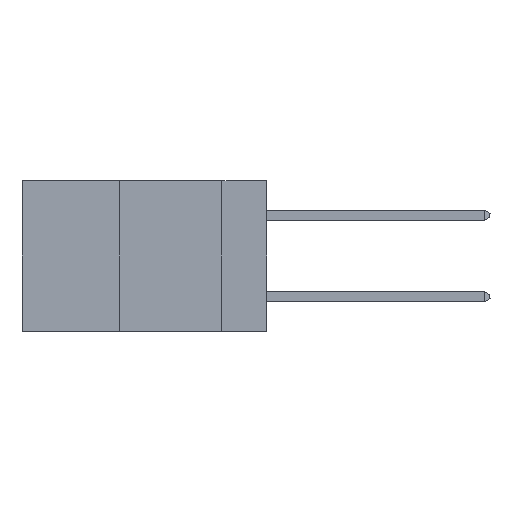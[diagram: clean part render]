
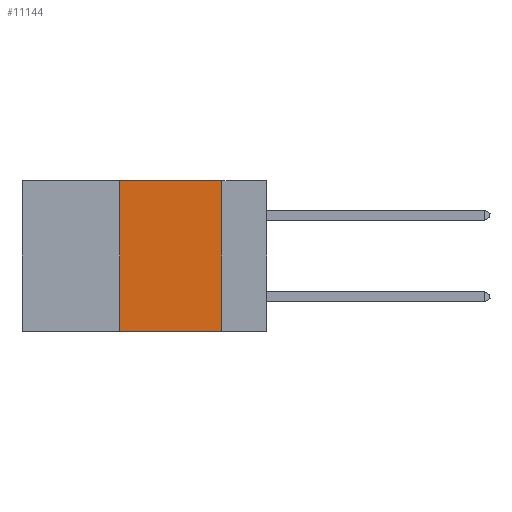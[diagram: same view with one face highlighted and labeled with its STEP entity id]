
A CAD part, left-side view. The second image highlights one B-rep face of the part: STEP entity #11144.
In plain terms, the highlighted planar face has unit normal (-1, 0, 0).
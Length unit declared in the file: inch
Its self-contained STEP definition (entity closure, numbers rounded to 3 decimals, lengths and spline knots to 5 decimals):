
#583 = DIRECTION ( 'NONE',  ( 0., 0., -1. ) ) ;
#2039 = LINE ( 'NONE', #22067, #15603 ) ;
#2174 = DIRECTION ( 'NONE',  ( 1., 0., 0. ) ) ;
#2341 = CARTESIAN_POINT ( 'NONE',  ( 0., 0.11, 0. ) ) ;
#3543 = AXIS2_PLACEMENT_3D ( 'NONE', #13882, #2174, #8664 ) ;
#5742 = LINE ( 'NONE', #2341, #22319 ) ;
#6015 = DIRECTION ( 'NONE',  ( 0., -1., 0. ) ) ;
#6436 = DIRECTION ( 'NONE',  ( 0., 0., 1. ) ) ;
#7558 = EDGE_CURVE ( 'NONE', #18047, #16710, #2039, .T. ) ;
#8325 = CARTESIAN_POINT ( 'NONE',  ( 0., 0.36, 0. ) ) ;
#8664 = DIRECTION ( 'NONE',  ( 0., 0., -1. ) ) ;
#9633 = PLANE ( 'NONE',  #3543 ) ;
#11144 = ADVANCED_FACE ( 'NONE', ( #20421 ), #9633, .F. ) ;
#12437 = DIRECTION ( 'NONE',  ( 0., -1., 0. ) ) ;
#13456 = LINE ( 'NONE', #8325, #18018 ) ;
#13805 = LINE ( 'NONE', #24127, #24475 ) ;
#13882 = CARTESIAN_POINT ( 'NONE',  ( 0., 0.6, 0. ) ) ;
#15603 = VECTOR ( 'NONE', #6015, 39.37008 ) ;
#15999 = CARTESIAN_POINT ( 'NONE',  ( 0., 0.36, -0.37 ) ) ;
#16649 = ORIENTED_EDGE ( 'NONE', *, *, #17976, .F. ) ;
#16710 = VERTEX_POINT ( 'NONE', #24221 ) ;
#16717 = EDGE_LOOP ( 'NONE', ( #24265, #18439, #16649, #22136 ) ) ;
#17144 = EDGE_CURVE ( 'NONE', #20373, #19151, #13805, .T. ) ;
#17976 = EDGE_CURVE ( 'NONE', #18047, #20373, #13456, .T. ) ;
#18018 = VECTOR ( 'NONE', #6436, 39.37008 ) ;
#18030 = EDGE_CURVE ( 'NONE', #19151, #16710, #5742, .T. ) ;
#18047 = VERTEX_POINT ( 'NONE', #15999 ) ;
#18439 = ORIENTED_EDGE ( 'NONE', *, *, #17144, .F. ) ;
#19151 = VERTEX_POINT ( 'NONE', #24826 ) ;
#20373 = VERTEX_POINT ( 'NONE', #24269 ) ;
#20421 = FACE_OUTER_BOUND ( 'NONE', #16717, .T. ) ;
#22067 = CARTESIAN_POINT ( 'NONE',  ( 0., 0.6, -0.37 ) ) ;
#22136 = ORIENTED_EDGE ( 'NONE', *, *, #7558, .T. ) ;
#22319 = VECTOR ( 'NONE', #583, 39.37008 ) ;
#24127 = CARTESIAN_POINT ( 'NONE',  ( 0., 0.6, 0. ) ) ;
#24221 = CARTESIAN_POINT ( 'NONE',  ( 0., 0.11, -0.37 ) ) ;
#24265 = ORIENTED_EDGE ( 'NONE', *, *, #18030, .F. ) ;
#24269 = CARTESIAN_POINT ( 'NONE',  ( 0., 0.36, 0. ) ) ;
#24475 = VECTOR ( 'NONE', #12437, 39.37008 ) ;
#24826 = CARTESIAN_POINT ( 'NONE',  ( 0., 0.11, 0. ) ) ;
